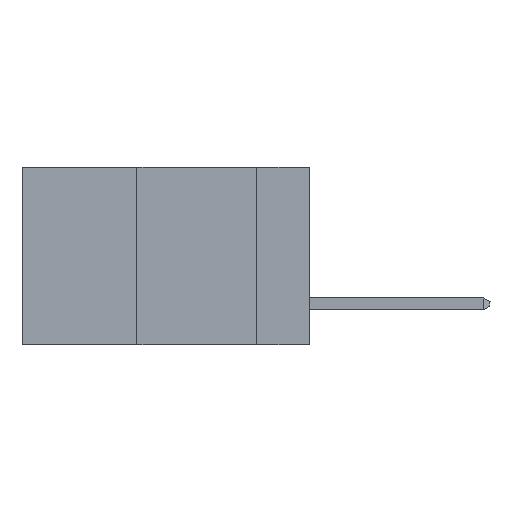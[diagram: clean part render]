
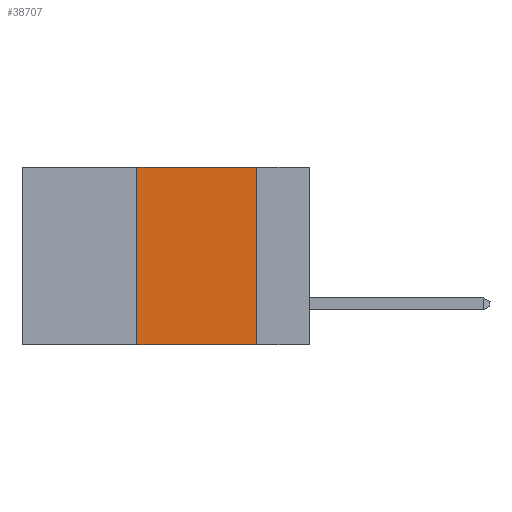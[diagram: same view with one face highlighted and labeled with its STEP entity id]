
A CAD part, left-side view. The second image highlights one B-rep face of the part: STEP entity #38707.
In plain terms, the highlighted planar face has unit normal (-1, 0, 0).
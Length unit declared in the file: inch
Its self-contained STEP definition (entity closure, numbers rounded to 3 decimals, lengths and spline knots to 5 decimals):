
#87 = DIRECTION ( 'NONE',  ( 0., 0., -1. ) ) ;
#237 = CARTESIAN_POINT ( 'NONE',  ( 0., 0.11, 0. ) ) ;
#813 = CARTESIAN_POINT ( 'NONE',  ( 0., 0.36, 0. ) ) ;
#1326 = LINE ( 'NONE', #813, #19809 ) ;
#2857 = EDGE_CURVE ( 'NONE', #20497, #42992, #3731, .T. ) ;
#3731 = LINE ( 'NONE', #5707, #11274 ) ;
#3883 = ORIENTED_EDGE ( 'NONE', *, *, #37437, .F. ) ;
#4581 = CARTESIAN_POINT ( 'NONE',  ( 0., 0.6, -0.37 ) ) ;
#5683 = FACE_OUTER_BOUND ( 'NONE', #32105, .T. ) ;
#5707 = CARTESIAN_POINT ( 'NONE',  ( 0., 0.6, 0. ) ) ;
#7038 = AXIS2_PLACEMENT_3D ( 'NONE', #35957, #10320, #24671 ) ;
#10320 = DIRECTION ( 'NONE',  ( 1., 0., 0. ) ) ;
#11274 = VECTOR ( 'NONE', #35540, 39.37008 ) ;
#11378 = LINE ( 'NONE', #237, #25228 ) ;
#14527 = ORIENTED_EDGE ( 'NONE', *, *, #34394, .F. ) ;
#18946 = EDGE_CURVE ( 'NONE', #19401, #47439, #39158, .T. ) ;
#19401 = VERTEX_POINT ( 'NONE', #39908 ) ;
#19809 = VECTOR ( 'NONE', #45167, 39.37008 ) ;
#20497 = VERTEX_POINT ( 'NONE', #28526 ) ;
#23805 = CARTESIAN_POINT ( 'NONE',  ( 0., 0.11, -0.37 ) ) ;
#24671 = DIRECTION ( 'NONE',  ( 0., 0., -1. ) ) ;
#25228 = VECTOR ( 'NONE', #87, 39.37008 ) ;
#26731 = DIRECTION ( 'NONE',  ( 0., -1., 0. ) ) ;
#28289 = ORIENTED_EDGE ( 'NONE', *, *, #2857, .F. ) ;
#28526 = CARTESIAN_POINT ( 'NONE',  ( 0., 0.36, 0. ) ) ;
#32105 = EDGE_LOOP ( 'NONE', ( #3883, #28289, #14527, #41504 ) ) ;
#32248 = PLANE ( 'NONE',  #7038 ) ;
#34394 = EDGE_CURVE ( 'NONE', #19401, #20497, #1326, .T. ) ;
#35540 = DIRECTION ( 'NONE',  ( 0., -1., 0. ) ) ;
#35957 = CARTESIAN_POINT ( 'NONE',  ( 0., 0.6, 0. ) ) ;
#37437 = EDGE_CURVE ( 'NONE', #42992, #47439, #11378, .T. ) ;
#38707 = ADVANCED_FACE ( 'NONE', ( #5683 ), #32248, .F. ) ;
#39158 = LINE ( 'NONE', #4581, #46105 ) ;
#39908 = CARTESIAN_POINT ( 'NONE',  ( 0., 0.36, -0.37 ) ) ;
#41504 = ORIENTED_EDGE ( 'NONE', *, *, #18946, .T. ) ;
#42136 = CARTESIAN_POINT ( 'NONE',  ( 0., 0.11, 0. ) ) ;
#42992 = VERTEX_POINT ( 'NONE', #42136 ) ;
#45167 = DIRECTION ( 'NONE',  ( 0., 0., 1. ) ) ;
#46105 = VECTOR ( 'NONE', #26731, 39.37008 ) ;
#47439 = VERTEX_POINT ( 'NONE', #23805 ) ;
